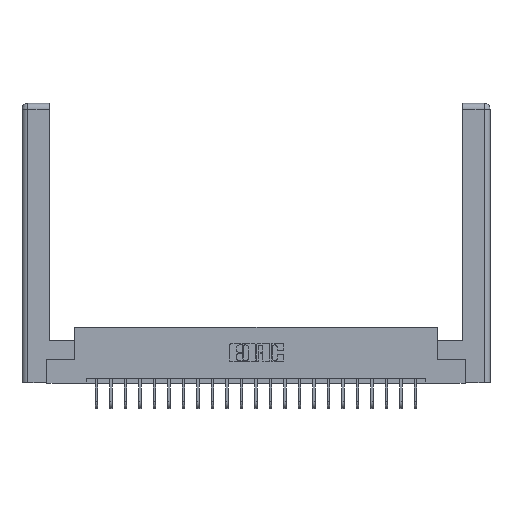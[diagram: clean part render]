
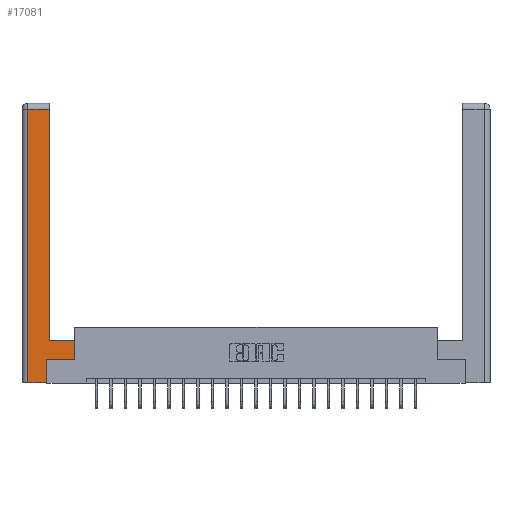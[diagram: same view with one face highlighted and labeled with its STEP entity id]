
A CAD part, top view. The second image highlights one B-rep face of the part: STEP entity #17081.
In plain terms, the highlighted planar face has unit normal (0, 0, 1).
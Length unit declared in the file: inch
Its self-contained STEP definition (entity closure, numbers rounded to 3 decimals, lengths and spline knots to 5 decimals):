
#4 = VECTOR ( 'NONE', #2964, 39.37008 ) ;
#42 = VECTOR ( 'NONE', #18999, 39.37008 ) ;
#100 = CARTESIAN_POINT ( 'NONE',  ( 0.565, 0.45, 0. ) ) ;
#357 = LINE ( 'NONE', #17534, #6559 ) ;
#439 = EDGE_CURVE ( 'NONE', #11506, #2037, #357, .T. ) ;
#1246 = VERTEX_POINT ( 'NONE', #4891 ) ;
#1332 = LINE ( 'NONE', #1604, #19613 ) ;
#1462 = DIRECTION ( 'NONE',  ( 1., 0., 0. ) ) ;
#1604 = CARTESIAN_POINT ( 'NONE',  ( 0.565, 0.45, 0. ) ) ;
#1996 = DIRECTION ( 'NONE',  ( -1., 0., 0. ) ) ;
#2037 = VERTEX_POINT ( 'NONE', #9976 ) ;
#2800 = EDGE_CURVE ( 'NONE', #1246, #11235, #2980, .T. ) ;
#2964 = DIRECTION ( 'NONE',  ( 0., 1., 0. ) ) ;
#2980 = LINE ( 'NONE', #7987, #9435 ) ;
#3196 = ORIENTED_EDGE ( 'NONE', *, *, #20748, .T. ) ;
#3711 = DIRECTION ( 'NONE',  ( 0., 1., 0. ) ) ;
#4572 = LINE ( 'NONE', #6428, #4 ) ;
#4613 = LINE ( 'NONE', #15454, #42 ) ;
#4891 = CARTESIAN_POINT ( 'NONE',  ( 0.265, 0.245, 0. ) ) ;
#5534 = CARTESIAN_POINT ( 'NONE',  ( 0.295, 2.94, 0. ) ) ;
#6420 = ORIENTED_EDGE ( 'NONE', *, *, #13256, .T. ) ;
#6428 = CARTESIAN_POINT ( 'NONE',  ( 0.265, 0.245, 0. ) ) ;
#6559 = VECTOR ( 'NONE', #1996, 39.37008 ) ;
#6986 = EDGE_CURVE ( 'NONE', #11235, #11506, #1332, .T. ) ;
#7121 = LINE ( 'NONE', #13290, #15712 ) ;
#7681 = CARTESIAN_POINT ( 'NONE',  ( 0.0615, 2.94, 0. ) ) ;
#7987 = CARTESIAN_POINT ( 'NONE',  ( 0.565, 0.245, 0. ) ) ;
#8642 = VERTEX_POINT ( 'NONE', #8816 ) ;
#8816 = CARTESIAN_POINT ( 'NONE',  ( 0.0615, 0., 0. ) ) ;
#9435 = VECTOR ( 'NONE', #14973, 39.37008 ) ;
#9976 = CARTESIAN_POINT ( 'NONE',  ( 0.295, 0.45, 0. ) ) ;
#10672 = FACE_OUTER_BOUND ( 'NONE', #21280, .T. ) ;
#11007 = ORIENTED_EDGE ( 'NONE', *, *, #439, .T. ) ;
#11011 = CARTESIAN_POINT ( 'NONE',  ( 0.565, 0.245, 0. ) ) ;
#11235 = VERTEX_POINT ( 'NONE', #11011 ) ;
#11238 = ORIENTED_EDGE ( 'NONE', *, *, #22263, .T. ) ;
#11288 = EDGE_CURVE ( 'NONE', #17806, #1246, #4572, .T. ) ;
#11506 = VERTEX_POINT ( 'NONE', #100 ) ;
#11540 = CARTESIAN_POINT ( 'NONE',  ( 0.265, 0., 0. ) ) ;
#12362 = CARTESIAN_POINT ( 'NONE',  ( 0.295, 3., 0. ) ) ;
#12498 = ORIENTED_EDGE ( 'NONE', *, *, #6986, .T. ) ;
#13256 = EDGE_CURVE ( 'NONE', #2037, #20261, #17485, .T. ) ;
#13290 = CARTESIAN_POINT ( 'NONE',  ( 0.265, 0., 0. ) ) ;
#13452 = LINE ( 'NONE', #21074, #13731 ) ;
#13731 = VECTOR ( 'NONE', #21145, 39.37008 ) ;
#13963 = ORIENTED_EDGE ( 'NONE', *, *, #11288, .T. ) ;
#14758 = PLANE ( 'NONE',  #19367 ) ;
#14973 = DIRECTION ( 'NONE',  ( 1., 0., 0. ) ) ;
#15454 = CARTESIAN_POINT ( 'NONE',  ( 0.0615, 0., 0. ) ) ;
#15712 = VECTOR ( 'NONE', #1462, 39.37008 ) ;
#15801 = DIRECTION ( 'NONE',  ( 0., 1., 0. ) ) ;
#16967 = VERTEX_POINT ( 'NONE', #7681 ) ;
#17081 = ADVANCED_FACE ( 'NONE', ( #10672 ), #14758, .F. ) ;
#17482 = ORIENTED_EDGE ( 'NONE', *, *, #2800, .T. ) ;
#17485 = LINE ( 'NONE', #12362, #18854 ) ;
#17534 = CARTESIAN_POINT ( 'NONE',  ( 0.295, 0.45, 0. ) ) ;
#17806 = VERTEX_POINT ( 'NONE', #11540 ) ;
#18164 = ORIENTED_EDGE ( 'NONE', *, *, #19419, .T. ) ;
#18408 = DIRECTION ( 'NONE',  ( 0., 0., -1. ) ) ;
#18854 = VECTOR ( 'NONE', #3711, 39.37008 ) ;
#18999 = DIRECTION ( 'NONE',  ( 0., -1., 0. ) ) ;
#19367 = AXIS2_PLACEMENT_3D ( 'NONE', #21653, #18408, #19921 ) ;
#19419 = EDGE_CURVE ( 'NONE', #8642, #17806, #7121, .T. ) ;
#19613 = VECTOR ( 'NONE', #15801, 39.37008 ) ;
#19921 = DIRECTION ( 'NONE',  ( -1., 0., 0. ) ) ;
#20261 = VERTEX_POINT ( 'NONE', #5534 ) ;
#20748 = EDGE_CURVE ( 'NONE', #16967, #8642, #4613, .T. ) ;
#21074 = CARTESIAN_POINT ( 'NONE',  ( 0.0615, 2.94, 0. ) ) ;
#21145 = DIRECTION ( 'NONE',  ( -1., 0., 0. ) ) ;
#21280 = EDGE_LOOP ( 'NONE', ( #6420, #11238, #3196, #18164, #13963, #17482, #12498, #11007 ) ) ;
#21653 = CARTESIAN_POINT ( 'NONE',  ( 0., 0., 0. ) ) ;
#22263 = EDGE_CURVE ( 'NONE', #20261, #16967, #13452, .T. ) ;
